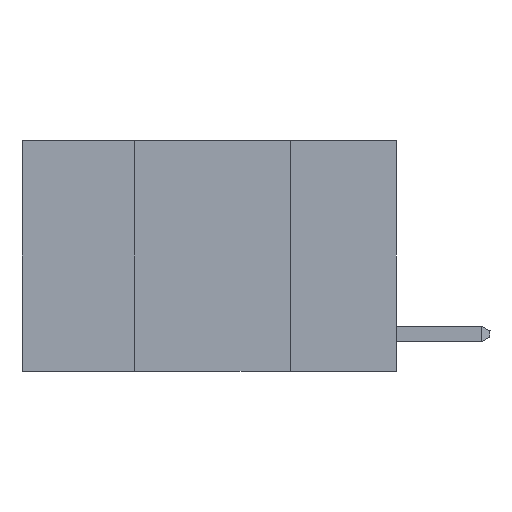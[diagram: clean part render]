
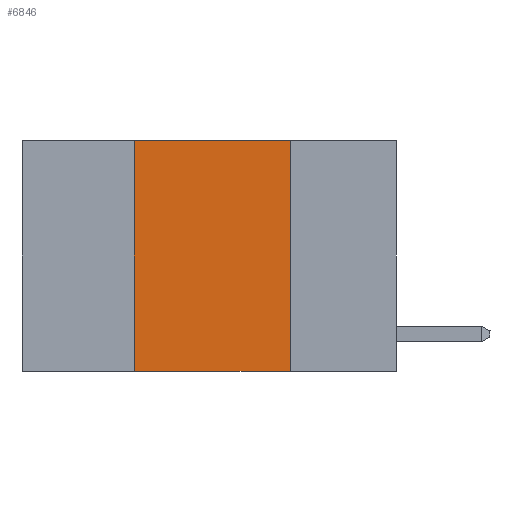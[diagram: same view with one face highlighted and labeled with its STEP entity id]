
A CAD part, left-side view. The second image highlights one B-rep face of the part: STEP entity #6846.
In plain terms, the highlighted planar face has unit normal (-1, 0, 0).
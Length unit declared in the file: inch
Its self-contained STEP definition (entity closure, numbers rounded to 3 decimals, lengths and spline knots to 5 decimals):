
#415 = ORIENTED_EDGE ( 'NONE', *, *, #7909, .F. ) ;
#1814 = VECTOR ( 'NONE', #14066, 39.37008 ) ;
#2126 = VECTOR ( 'NONE', #4168, 39.37008 ) ;
#2779 = LINE ( 'NONE', #10248, #2126 ) ;
#3031 = VECTOR ( 'NONE', #21307, 39.37008 ) ;
#4168 = DIRECTION ( 'NONE',  ( 0., -1., 0. ) ) ;
#5194 = EDGE_CURVE ( 'NONE', #26090, #25077, #6591, .T. ) ;
#5950 = ORIENTED_EDGE ( 'NONE', *, *, #5194, .T. ) ;
#6527 = EDGE_CURVE ( 'NONE', #26090, #22701, #18014, .T. ) ;
#6591 = LINE ( 'NONE', #26274, #1814 ) ;
#6846 = ADVANCED_FACE ( 'NONE', ( #24737 ), #18238, .F. ) ;
#7909 = EDGE_CURVE ( 'NONE', #12314, #25077, #26239, .T. ) ;
#8080 = DIRECTION ( 'NONE',  ( 1., 0., 0. ) ) ;
#8407 = EDGE_LOOP ( 'NONE', ( #415, #19773, #19059, #5950 ) ) ;
#10248 = CARTESIAN_POINT ( 'NONE',  ( 0., 0.6, 0. ) ) ;
#11425 = DIRECTION ( 'NONE',  ( 0., 0., -1. ) ) ;
#12314 = VERTEX_POINT ( 'NONE', #13369 ) ;
#13369 = CARTESIAN_POINT ( 'NONE',  ( 0., 0.17, 0. ) ) ;
#14066 = DIRECTION ( 'NONE',  ( 0., -1., 0. ) ) ;
#18014 = LINE ( 'NONE', #19236, #3031 ) ;
#18238 = PLANE ( 'NONE',  #23182 ) ;
#19059 = ORIENTED_EDGE ( 'NONE', *, *, #6527, .F. ) ;
#19236 = CARTESIAN_POINT ( 'NONE',  ( 0., 0.42, 0. ) ) ;
#19773 = ORIENTED_EDGE ( 'NONE', *, *, #26410, .F. ) ;
#20286 = CARTESIAN_POINT ( 'NONE',  ( 0., 0.6, 0. ) ) ;
#21307 = DIRECTION ( 'NONE',  ( 0., 0., 1. ) ) ;
#21604 = CARTESIAN_POINT ( 'NONE',  ( 0., 0.42, -0.37 ) ) ;
#22368 = DIRECTION ( 'NONE',  ( 0., 0., -1. ) ) ;
#22701 = VERTEX_POINT ( 'NONE', #25192 ) ;
#23182 = AXIS2_PLACEMENT_3D ( 'NONE', #20286, #8080, #22368 ) ;
#23403 = VECTOR ( 'NONE', #11425, 39.37008 ) ;
#23678 = CARTESIAN_POINT ( 'NONE',  ( 0., 0.17, 0. ) ) ;
#24245 = CARTESIAN_POINT ( 'NONE',  ( 0., 0.17, -0.37 ) ) ;
#24737 = FACE_OUTER_BOUND ( 'NONE', #8407, .T. ) ;
#25077 = VERTEX_POINT ( 'NONE', #24245 ) ;
#25192 = CARTESIAN_POINT ( 'NONE',  ( 0., 0.42, 0. ) ) ;
#26090 = VERTEX_POINT ( 'NONE', #21604 ) ;
#26239 = LINE ( 'NONE', #23678, #23403 ) ;
#26274 = CARTESIAN_POINT ( 'NONE',  ( 0., 0.6, -0.37 ) ) ;
#26410 = EDGE_CURVE ( 'NONE', #22701, #12314, #2779, .T. ) ;
